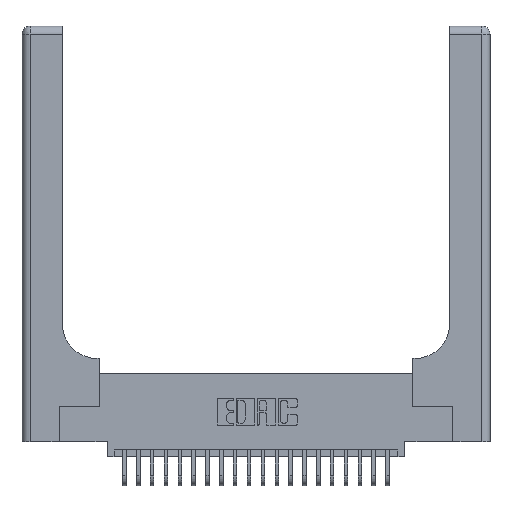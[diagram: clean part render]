
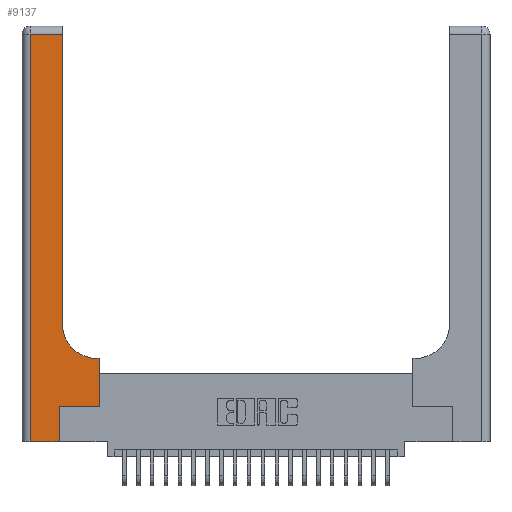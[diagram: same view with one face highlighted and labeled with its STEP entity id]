
A CAD part, top view. The second image highlights one B-rep face of the part: STEP entity #9137.
In plain terms, the highlighted planar face has unit normal (0, 0, 1).
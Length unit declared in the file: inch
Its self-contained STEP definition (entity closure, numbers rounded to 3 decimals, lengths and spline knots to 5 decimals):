
#404 = EDGE_CURVE ( 'NONE', #12892, #8088, #20060, .T. ) ;
#453 = VECTOR ( 'NONE', #10834, 39.37008 ) ;
#515 = DIRECTION ( 'NONE',  ( 0., -1., 0. ) ) ;
#724 = ORIENTED_EDGE ( 'NONE', *, *, #5332, .T. ) ;
#978 = CARTESIAN_POINT ( 'NONE',  ( 0.2915, 0.6, 0.37 ) ) ;
#1114 = ORIENTED_EDGE ( 'NONE', *, *, #19859, .T. ) ;
#1253 = CARTESIAN_POINT ( 'NONE',  ( 0.5585, 0.6, 0.37 ) ) ;
#2145 = CARTESIAN_POINT ( 'NONE',  ( 0.2915, 2.94, 0.37 ) ) ;
#3216 = VECTOR ( 'NONE', #9489, 39.37008 ) ;
#5244 = VECTOR ( 'NONE', #13653, 39.37008 ) ;
#5332 = EDGE_CURVE ( 'NONE', #23151, #18259, #8672, .T. ) ;
#5444 = DIRECTION ( 'NONE',  ( -1., 0., 0. ) ) ;
#5470 = LINE ( 'NONE', #978, #19962 ) ;
#5869 = LINE ( 'NONE', #23691, #5244 ) ;
#6250 = DIRECTION ( 'NONE',  ( 1., 0., 0. ) ) ;
#6298 = EDGE_CURVE ( 'NONE', #7382, #11109, #14246, .T. ) ;
#6371 = DIRECTION ( 'NONE',  ( 1., 0., 0. ) ) ;
#6602 = CARTESIAN_POINT ( 'NONE',  ( 0.269, 0., 0.37 ) ) ;
#7065 = CARTESIAN_POINT ( 'NONE',  ( 0., 3., 0.37 ) ) ;
#7348 = VECTOR ( 'NONE', #25102, 39.37008 ) ;
#7382 = VERTEX_POINT ( 'NONE', #9036 ) ;
#7902 = ORIENTED_EDGE ( 'NONE', *, *, #17131, .T. ) ;
#8088 = VERTEX_POINT ( 'NONE', #11017 ) ;
#8672 = CIRCLE ( 'NONE', #18365, 0.25 ) ;
#9034 = CARTESIAN_POINT ( 'NONE',  ( 0.06, 0., 0.37 ) ) ;
#9036 = CARTESIAN_POINT ( 'NONE',  ( 0.5585, 0.25, 0.37 ) ) ;
#9044 = DIRECTION ( 'NONE',  ( 0., 0., -1. ) ) ;
#9137 = ADVANCED_FACE ( 'NONE', ( #17840 ), #20682, .F. ) ;
#9489 = DIRECTION ( 'NONE',  ( 0., 1., 0. ) ) ;
#10402 = CARTESIAN_POINT ( 'NONE',  ( 0.06, 3., 0.37 ) ) ;
#10520 = VERTEX_POINT ( 'NONE', #9034 ) ;
#10731 = LINE ( 'NONE', #20972, #453 ) ;
#10834 = DIRECTION ( 'NONE',  ( 0., 1., 0. ) ) ;
#11017 = CARTESIAN_POINT ( 'NONE',  ( 0.06, 2.94, 0.37 ) ) ;
#11058 = EDGE_CURVE ( 'NONE', #8088, #10520, #24825, .T. ) ;
#11109 = VERTEX_POINT ( 'NONE', #1253 ) ;
#11620 = ORIENTED_EDGE ( 'NONE', *, *, #404, .T. ) ;
#11669 = ORIENTED_EDGE ( 'NONE', *, *, #11058, .T. ) ;
#11673 = ORIENTED_EDGE ( 'NONE', *, *, #6298, .T. ) ;
#11766 = CARTESIAN_POINT ( 'NONE',  ( 0.2915, 0.85, 0.37 ) ) ;
#11960 = VECTOR ( 'NONE', #6371, 39.37008 ) ;
#12892 = VERTEX_POINT ( 'NONE', #2145 ) ;
#13040 = EDGE_CURVE ( 'NONE', #11109, #23151, #5470, .T. ) ;
#13653 = DIRECTION ( 'NONE',  ( 0., 1., 0. ) ) ;
#14246 = LINE ( 'NONE', #20343, #3216 ) ;
#14534 = ORIENTED_EDGE ( 'NONE', *, *, #21966, .T. ) ;
#14916 = EDGE_CURVE ( 'NONE', #10520, #19542, #24737, .T. ) ;
#17131 = EDGE_CURVE ( 'NONE', #18925, #7382, #21249, .T. ) ;
#17840 = FACE_OUTER_BOUND ( 'NONE', #24996, .T. ) ;
#18203 = CARTESIAN_POINT ( 'NONE',  ( 0.269, 0.25, 0.37 ) ) ;
#18259 = VERTEX_POINT ( 'NONE', #11766 ) ;
#18365 = AXIS2_PLACEMENT_3D ( 'NONE', #21474, #19574, #6250 ) ;
#18381 = CARTESIAN_POINT ( 'NONE',  ( 0., 0., 0.37 ) ) ;
#18925 = VERTEX_POINT ( 'NONE', #22241 ) ;
#19533 = AXIS2_PLACEMENT_3D ( 'NONE', #7065, #9044, #20855 ) ;
#19542 = VERTEX_POINT ( 'NONE', #6602 ) ;
#19574 = DIRECTION ( 'NONE',  ( 0., 0., -1. ) ) ;
#19650 = CARTESIAN_POINT ( 'NONE',  ( 0.5415, 0.6, 0.37 ) ) ;
#19658 = ORIENTED_EDGE ( 'NONE', *, *, #14916, .T. ) ;
#19859 = EDGE_CURVE ( 'NONE', #19542, #18925, #5869, .T. ) ;
#19962 = VECTOR ( 'NONE', #5444, 39.37008 ) ;
#20060 = LINE ( 'NONE', #25316, #7348 ) ;
#20343 = CARTESIAN_POINT ( 'NONE',  ( 0.5585, 0.25, 0.37 ) ) ;
#20682 = PLANE ( 'NONE',  #19533 ) ;
#20855 = DIRECTION ( 'NONE',  ( -1., 0., 0. ) ) ;
#20972 = CARTESIAN_POINT ( 'NONE',  ( 0.2915, 3., 0.37 ) ) ;
#21249 = LINE ( 'NONE', #18203, #11960 ) ;
#21474 = CARTESIAN_POINT ( 'NONE',  ( 0.5415, 0.85, 0.37 ) ) ;
#21966 = EDGE_CURVE ( 'NONE', #18259, #12892, #10731, .T. ) ;
#22241 = CARTESIAN_POINT ( 'NONE',  ( 0.269, 0.25, 0.37 ) ) ;
#22872 = VECTOR ( 'NONE', #24265, 39.37008 ) ;
#23151 = VERTEX_POINT ( 'NONE', #19650 ) ;
#23691 = CARTESIAN_POINT ( 'NONE',  ( 0.269, 0., 0.37 ) ) ;
#23917 = VECTOR ( 'NONE', #515, 39.37008 ) ;
#24265 = DIRECTION ( 'NONE',  ( 1., 0., 0. ) ) ;
#24281 = ORIENTED_EDGE ( 'NONE', *, *, #13040, .T. ) ;
#24737 = LINE ( 'NONE', #18381, #22872 ) ;
#24825 = LINE ( 'NONE', #10402, #23917 ) ;
#24996 = EDGE_LOOP ( 'NONE', ( #14534, #11620, #11669, #19658, #1114, #7902, #11673, #24281, #724 ) ) ;
#25102 = DIRECTION ( 'NONE',  ( -1., 0., 0. ) ) ;
#25316 = CARTESIAN_POINT ( 'NONE',  ( 0., 2.94, 0.37 ) ) ;
